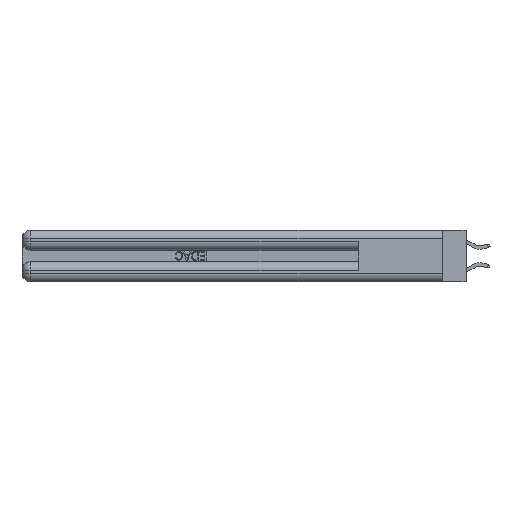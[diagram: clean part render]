
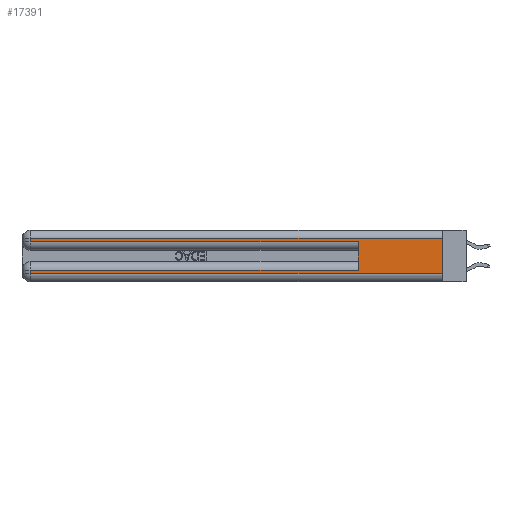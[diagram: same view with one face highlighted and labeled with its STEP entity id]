
A CAD part, left-side view. The second image highlights one B-rep face of the part: STEP entity #17391.
In plain terms, the highlighted planar face has unit normal (-1, 0, 0).
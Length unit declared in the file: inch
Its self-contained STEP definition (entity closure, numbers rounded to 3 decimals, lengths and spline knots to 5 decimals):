
#183 = ORIENTED_EDGE ( 'NONE', *, *, #6346, .T. ) ;
#246 = CARTESIAN_POINT ( 'NONE',  ( 0., 2.94, 0.31 ) ) ;
#333 = CARTESIAN_POINT ( 'NONE',  ( 0., 0., 0.06 ) ) ;
#493 = ORIENTED_EDGE ( 'NONE', *, *, #9114, .T. ) ;
#565 = CARTESIAN_POINT ( 'NONE',  ( 0., 0., 0.37 ) ) ;
#923 = ORIENTED_EDGE ( 'NONE', *, *, #11004, .T. ) ;
#1009 = VECTOR ( 'NONE', #20524, 39.37008 ) ;
#1844 = CARTESIAN_POINT ( 'NONE',  ( 0., 2.94, 0.085 ) ) ;
#2465 = LINE ( 'NONE', #333, #15061 ) ;
#2872 = DIRECTION ( 'NONE',  ( 0., -1., 0. ) ) ;
#3870 = EDGE_LOOP ( 'NONE', ( #17408, #11587, #25621, #13129, #26410, #183, #493, #923 ) ) ;
#4069 = VECTOR ( 'NONE', #12576, 39.37008 ) ;
#4943 = VECTOR ( 'NONE', #11054, 39.37008 ) ;
#5634 = DIRECTION ( 'NONE',  ( 0., 0., -1. ) ) ;
#6346 = EDGE_CURVE ( 'NONE', #11865, #12102, #24133, .T. ) ;
#6920 = VECTOR ( 'NONE', #12136, 39.37008 ) ;
#7231 = CARTESIAN_POINT ( 'NONE',  ( 0., 2.94, 0.37 ) ) ;
#7714 = LINE ( 'NONE', #14645, #6920 ) ;
#7820 = FACE_OUTER_BOUND ( 'NONE', #3870, .T. ) ;
#8706 = CARTESIAN_POINT ( 'NONE',  ( 0., 2.94, 0.285 ) ) ;
#9096 = VECTOR ( 'NONE', #16585, 39.37008 ) ;
#9114 = EDGE_CURVE ( 'NONE', #12102, #26393, #7714, .T. ) ;
#10094 = CARTESIAN_POINT ( 'NONE',  ( 0., 0.6, 0.145 ) ) ;
#10901 = AXIS2_PLACEMENT_3D ( 'NONE', #565, #20621, #5634 ) ;
#11004 = EDGE_CURVE ( 'NONE', #26393, #16197, #2465, .T. ) ;
#11054 = DIRECTION ( 'NONE',  ( 0., 1., 0. ) ) ;
#11587 = ORIENTED_EDGE ( 'NONE', *, *, #28398, .T. ) ;
#11865 = VERTEX_POINT ( 'NONE', #23320 ) ;
#12102 = VERTEX_POINT ( 'NONE', #1844 ) ;
#12136 = DIRECTION ( 'NONE',  ( 0., 0., -1. ) ) ;
#12576 = DIRECTION ( 'NONE',  ( 0., 0., 1. ) ) ;
#13129 = ORIENTED_EDGE ( 'NONE', *, *, #15607, .T. ) ;
#14645 = CARTESIAN_POINT ( 'NONE',  ( 0., 2.94, 0.37 ) ) ;
#15061 = VECTOR ( 'NONE', #2872, 39.37008 ) ;
#15098 = CARTESIAN_POINT ( 'NONE',  ( 0., 0., 0.37 ) ) ;
#15607 = EDGE_CURVE ( 'NONE', #32014, #22594, #16489, .T. ) ;
#16197 = VERTEX_POINT ( 'NONE', #18617 ) ;
#16489 = LINE ( 'NONE', #31585, #9096 ) ;
#16585 = DIRECTION ( 'NONE',  ( 0., -1., 0. ) ) ;
#17176 = CARTESIAN_POINT ( 'NONE',  ( 0., 0.6, 0.285 ) ) ;
#17391 = ADVANCED_FACE ( 'NONE', ( #7820 ), #18111, .F. ) ;
#17408 = ORIENTED_EDGE ( 'NONE', *, *, #21269, .F. ) ;
#18111 = PLANE ( 'NONE',  #10901 ) ;
#18157 = CARTESIAN_POINT ( 'NONE',  ( 0., 0., 0.31 ) ) ;
#18617 = CARTESIAN_POINT ( 'NONE',  ( 0., 0., 0.06 ) ) ;
#19359 = EDGE_CURVE ( 'NONE', #31197, #32014, #22126, .T. ) ;
#19984 = EDGE_CURVE ( 'NONE', #11865, #22594, #24838, .T. ) ;
#20524 = DIRECTION ( 'NONE',  ( 0., 1., 0. ) ) ;
#20621 = DIRECTION ( 'NONE',  ( 1., 0., 0. ) ) ;
#21269 = EDGE_CURVE ( 'NONE', #25916, #16197, #30876, .T. ) ;
#21788 = LINE ( 'NONE', #27994, #1009 ) ;
#22126 = LINE ( 'NONE', #7231, #22907 ) ;
#22594 = VERTEX_POINT ( 'NONE', #17176 ) ;
#22907 = VECTOR ( 'NONE', #27245, 39.37008 ) ;
#23320 = CARTESIAN_POINT ( 'NONE',  ( 0., 0.6, 0.085 ) ) ;
#24133 = LINE ( 'NONE', #25647, #4943 ) ;
#24838 = LINE ( 'NONE', #10094, #4069 ) ;
#25621 = ORIENTED_EDGE ( 'NONE', *, *, #19359, .T. ) ;
#25647 = CARTESIAN_POINT ( 'NONE',  ( 0., 0., 0.085 ) ) ;
#25916 = VERTEX_POINT ( 'NONE', #18157 ) ;
#26393 = VERTEX_POINT ( 'NONE', #32060 ) ;
#26410 = ORIENTED_EDGE ( 'NONE', *, *, #19984, .F. ) ;
#27245 = DIRECTION ( 'NONE',  ( 0., 0., -1. ) ) ;
#27560 = DIRECTION ( 'NONE',  ( 0., 0., -1. ) ) ;
#27994 = CARTESIAN_POINT ( 'NONE',  ( 0., 0., 0.31 ) ) ;
#28398 = EDGE_CURVE ( 'NONE', #25916, #31197, #21788, .T. ) ;
#30102 = VECTOR ( 'NONE', #27560, 39.37008 ) ;
#30876 = LINE ( 'NONE', #15098, #30102 ) ;
#31197 = VERTEX_POINT ( 'NONE', #246 ) ;
#31585 = CARTESIAN_POINT ( 'NONE',  ( 0., 0., 0.285 ) ) ;
#32014 = VERTEX_POINT ( 'NONE', #8706 ) ;
#32060 = CARTESIAN_POINT ( 'NONE',  ( 0., 2.94, 0.06 ) ) ;
